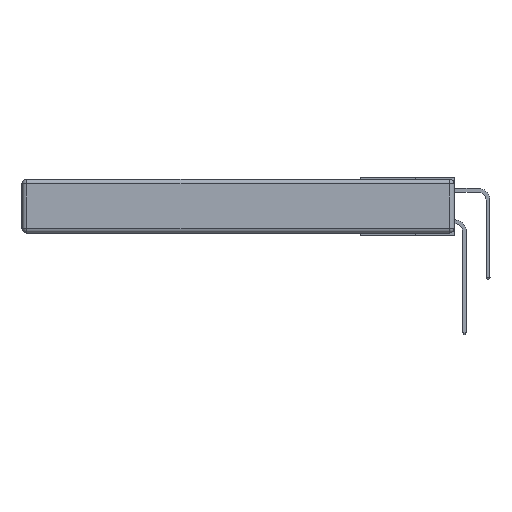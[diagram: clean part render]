
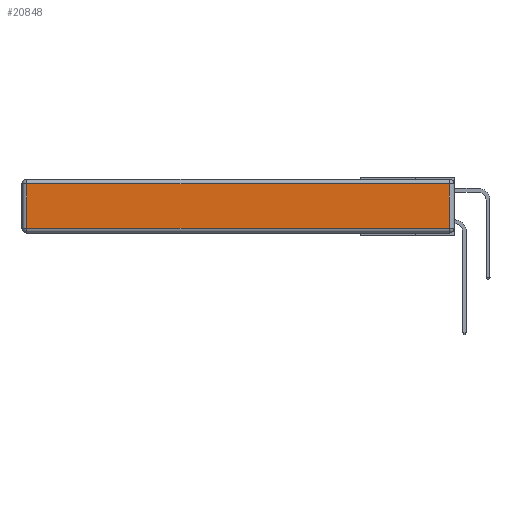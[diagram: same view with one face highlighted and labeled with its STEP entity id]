
A CAD part, left-side view. The second image highlights one B-rep face of the part: STEP entity #20848.
In plain terms, the highlighted planar face has unit normal (-1, 0, 0).
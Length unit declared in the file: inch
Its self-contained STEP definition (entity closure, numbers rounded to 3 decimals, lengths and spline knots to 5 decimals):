
#97 = LINE ( 'NONE', #336, #3210 ) ;
#336 = CARTESIAN_POINT ( 'NONE',  ( 0., 2.72, -0.343 ) ) ;
#915 = LINE ( 'NONE', #23282, #2620 ) ;
#1613 = FACE_OUTER_BOUND ( 'NONE', #16435, .T. ) ;
#2620 = VECTOR ( 'NONE', #12357, 39.37008 ) ;
#2879 = DIRECTION ( 'NONE',  ( 0., 0., 1. ) ) ;
#2932 = VERTEX_POINT ( 'NONE', #20555 ) ;
#3210 = VECTOR ( 'NONE', #13053, 39.37008 ) ;
#4235 = EDGE_CURVE ( 'NONE', #5281, #5968, #97, .T. ) ;
#5281 = VERTEX_POINT ( 'NONE', #9721 ) ;
#5968 = VERTEX_POINT ( 'NONE', #14169 ) ;
#7826 = ORIENTED_EDGE ( 'NONE', *, *, #4235, .T. ) ;
#7849 = ORIENTED_EDGE ( 'NONE', *, *, #14577, .T. ) ;
#8063 = CARTESIAN_POINT ( 'NONE',  ( 0., 0.03, -0.343 ) ) ;
#9721 = CARTESIAN_POINT ( 'NONE',  ( 0., 2.72, -0.03 ) ) ;
#9872 = DIRECTION ( 'NONE',  ( 0., 0., 1. ) ) ;
#9939 = EDGE_CURVE ( 'NONE', #10674, #2932, #16612, .T. ) ;
#10674 = VERTEX_POINT ( 'NONE', #13359 ) ;
#11456 = DIRECTION ( 'NONE',  ( 0., 1., 0. ) ) ;
#11768 = CARTESIAN_POINT ( 'NONE',  ( 0., 0., -0.343 ) ) ;
#12357 = DIRECTION ( 'NONE',  ( 0., -1., 0. ) ) ;
#13053 = DIRECTION ( 'NONE',  ( 0., 0., -1. ) ) ;
#13359 = CARTESIAN_POINT ( 'NONE',  ( 0., 0.03, -0.313 ) ) ;
#14169 = CARTESIAN_POINT ( 'NONE',  ( 0., 2.72, -0.313 ) ) ;
#14537 = LINE ( 'NONE', #20521, #21059 ) ;
#14577 = EDGE_CURVE ( 'NONE', #2932, #5281, #14537, .T. ) ;
#15225 = EDGE_CURVE ( 'NONE', #5968, #10674, #915, .T. ) ;
#15983 = AXIS2_PLACEMENT_3D ( 'NONE', #11768, #19094, #2879 ) ;
#16435 = EDGE_LOOP ( 'NONE', ( #20935, #20583, #7849, #7826 ) ) ;
#16612 = LINE ( 'NONE', #8063, #18613 ) ;
#18613 = VECTOR ( 'NONE', #9872, 39.37008 ) ;
#19094 = DIRECTION ( 'NONE',  ( -1., 0., 0. ) ) ;
#20521 = CARTESIAN_POINT ( 'NONE',  ( 0., 2.75, -0.03 ) ) ;
#20555 = CARTESIAN_POINT ( 'NONE',  ( 0., 0.03, -0.03 ) ) ;
#20583 = ORIENTED_EDGE ( 'NONE', *, *, #9939, .T. ) ;
#20756 = PLANE ( 'NONE',  #15983 ) ;
#20848 = ADVANCED_FACE ( 'NONE', ( #1613 ), #20756, .T. ) ;
#20935 = ORIENTED_EDGE ( 'NONE', *, *, #15225, .T. ) ;
#21059 = VECTOR ( 'NONE', #11456, 39.37008 ) ;
#23282 = CARTESIAN_POINT ( 'NONE',  ( 0., 0., -0.313 ) ) ;
